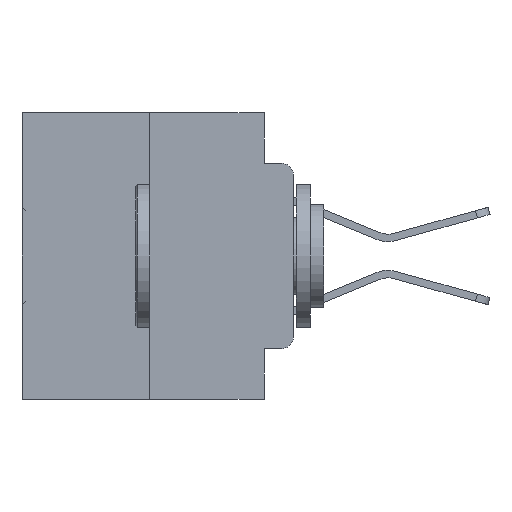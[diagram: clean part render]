
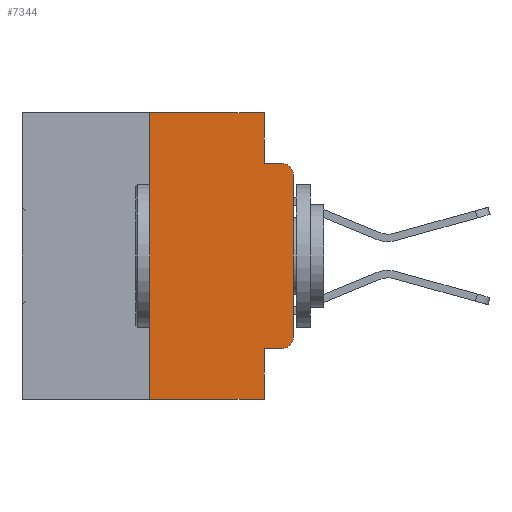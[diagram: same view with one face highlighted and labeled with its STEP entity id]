
A CAD part, left-side view. The second image highlights one B-rep face of the part: STEP entity #7344.
In plain terms, the highlighted planar face has unit normal (-1, 0, 0).
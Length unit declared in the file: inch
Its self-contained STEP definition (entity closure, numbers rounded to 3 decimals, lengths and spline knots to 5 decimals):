
#175 = EDGE_CURVE ( 'NONE', #24864, #2652, #18759, .T. ) ;
#253 = EDGE_CURVE ( 'NONE', #2652, #20397, #9630, .T. ) ;
#438 = CARTESIAN_POINT ( 'NONE',  ( 0., 0.051, -0.0885 ) ) ;
#576 = CARTESIAN_POINT ( 'NONE',  ( 0., 0.051, 0. ) ) ;
#759 = PLANE ( 'NONE',  #2581 ) ;
#1670 = VERTEX_POINT ( 'NONE', #30321 ) ;
#1920 = ORIENTED_EDGE ( 'NONE', *, *, #18589, .T. ) ;
#2013 = DIRECTION ( 'NONE',  ( 0., 0., -1. ) ) ;
#2068 = CARTESIAN_POINT ( 'NONE',  ( 0., 0.25, 0. ) ) ;
#2276 = CARTESIAN_POINT ( 'NONE',  ( 0., 0.02, -0.4115 ) ) ;
#2544 = VECTOR ( 'NONE', #8177, 39.37008 ) ;
#2581 = AXIS2_PLACEMENT_3D ( 'NONE', #8511, #15895, #5812 ) ;
#2652 = VERTEX_POINT ( 'NONE', #10949 ) ;
#3307 = VECTOR ( 'NONE', #26585, 39.37008 ) ;
#4501 = VERTEX_POINT ( 'NONE', #12056 ) ;
#4738 = VECTOR ( 'NONE', #5002, 39.37008 ) ;
#4753 = EDGE_CURVE ( 'NONE', #4501, #22494, #8664, .T. ) ;
#5002 = DIRECTION ( 'NONE',  ( 0., -1., 0. ) ) ;
#5324 = LINE ( 'NONE', #15572, #4738 ) ;
#5365 = DIRECTION ( 'NONE',  ( 0., -1., 0. ) ) ;
#5481 = CARTESIAN_POINT ( 'NONE',  ( 0., 0.051, -0.4115 ) ) ;
#5764 = LINE ( 'NONE', #31781, #31315 ) ;
#5812 = DIRECTION ( 'NONE',  ( 0., 0., -1. ) ) ;
#6487 = CARTESIAN_POINT ( 'NONE',  ( 0., 0.25, 0. ) ) ;
#7344 = ADVANCED_FACE ( 'NONE', ( #28811 ), #759, .F. ) ;
#7726 = EDGE_CURVE ( 'NONE', #24086, #4501, #5324, .T. ) ;
#8177 = DIRECTION ( 'NONE',  ( 0., 0., 1. ) ) ;
#8352 = CARTESIAN_POINT ( 'NONE',  ( 0., 0., 0. ) ) ;
#8430 = CARTESIAN_POINT ( 'NONE',  ( 0., 0.02, -0.0885 ) ) ;
#8511 = CARTESIAN_POINT ( 'NONE',  ( 0., 0.473, 0. ) ) ;
#8664 = LINE ( 'NONE', #576, #22919 ) ;
#9367 = DIRECTION ( 'NONE',  ( 0., 0., -1. ) ) ;
#9630 = CIRCLE ( 'NONE', #31566, 0.02 ) ;
#9819 = VECTOR ( 'NONE', #5365, 39.37008 ) ;
#10439 = LINE ( 'NONE', #13259, #24296 ) ;
#10949 = CARTESIAN_POINT ( 'NONE',  ( 0., 0., -0.1085 ) ) ;
#11005 = DIRECTION ( 'NONE',  ( 0., 0., -1. ) ) ;
#11677 = DIRECTION ( 'NONE',  ( 0., 0., 1. ) ) ;
#11937 = VERTEX_POINT ( 'NONE', #5481 ) ;
#12056 = CARTESIAN_POINT ( 'NONE',  ( 0., 0.051, 0. ) ) ;
#12322 = CARTESIAN_POINT ( 'NONE',  ( 0., 0., -0.3915 ) ) ;
#12771 = DIRECTION ( 'NONE',  ( 0., -1., 0. ) ) ;
#13259 = CARTESIAN_POINT ( 'NONE',  ( 0., 0.051, -0.4115 ) ) ;
#13326 = ORIENTED_EDGE ( 'NONE', *, *, #7726, .F. ) ;
#13506 = LINE ( 'NONE', #31626, #3307 ) ;
#14018 = EDGE_CURVE ( 'NONE', #19169, #24086, #22564, .T. ) ;
#14299 = DIRECTION ( 'NONE',  ( -1., 0., 0. ) ) ;
#15572 = CARTESIAN_POINT ( 'NONE',  ( 0., 0.473, 0. ) ) ;
#15895 = DIRECTION ( 'NONE',  ( 1., 0., 0. ) ) ;
#16673 = EDGE_CURVE ( 'NONE', #11937, #1670, #5764, .T. ) ;
#17281 = EDGE_LOOP ( 'NONE', ( #30604, #31791, #18895, #23399, #13326, #21141, #28753, #22135, #27147, #1920 ) ) ;
#18476 = LINE ( 'NONE', #26006, #9819 ) ;
#18589 = EDGE_CURVE ( 'NONE', #22870, #24864, #28412, .T. ) ;
#18759 = LINE ( 'NONE', #8352, #2544 ) ;
#18895 = ORIENTED_EDGE ( 'NONE', *, *, #32709, .F. ) ;
#19169 = VERTEX_POINT ( 'NONE', #20621 ) ;
#20397 = VERTEX_POINT ( 'NONE', #8430 ) ;
#20621 = CARTESIAN_POINT ( 'NONE',  ( 0., 0.25, -0.5 ) ) ;
#21141 = ORIENTED_EDGE ( 'NONE', *, *, #14018, .F. ) ;
#22034 = EDGE_CURVE ( 'NONE', #11937, #22870, #10439, .T. ) ;
#22135 = ORIENTED_EDGE ( 'NONE', *, *, #16673, .F. ) ;
#22494 = VERTEX_POINT ( 'NONE', #438 ) ;
#22564 = LINE ( 'NONE', #2068, #25795 ) ;
#22870 = VERTEX_POINT ( 'NONE', #2276 ) ;
#22919 = VECTOR ( 'NONE', #31142, 39.37008 ) ;
#23399 = ORIENTED_EDGE ( 'NONE', *, *, #4753, .F. ) ;
#24086 = VERTEX_POINT ( 'NONE', #6487 ) ;
#24296 = VECTOR ( 'NONE', #12771, 39.37008 ) ;
#24864 = VERTEX_POINT ( 'NONE', #12322 ) ;
#25795 = VECTOR ( 'NONE', #11677, 39.37008 ) ;
#26006 = CARTESIAN_POINT ( 'NONE',  ( 0., 0.051, -0.0885 ) ) ;
#26585 = DIRECTION ( 'NONE',  ( 0., -1., 0. ) ) ;
#26782 = DIRECTION ( 'NONE',  ( -1., 0., 0. ) ) ;
#27147 = ORIENTED_EDGE ( 'NONE', *, *, #22034, .T. ) ;
#28412 = CIRCLE ( 'NONE', #29470, 0.02 ) ;
#28753 = ORIENTED_EDGE ( 'NONE', *, *, #31816, .T. ) ;
#28811 = FACE_OUTER_BOUND ( 'NONE', #17281, .T. ) ;
#29470 = AXIS2_PLACEMENT_3D ( 'NONE', #32582, #14299, #2013 ) ;
#30321 = CARTESIAN_POINT ( 'NONE',  ( 0., 0.051, -0.5 ) ) ;
#30604 = ORIENTED_EDGE ( 'NONE', *, *, #175, .T. ) ;
#31142 = DIRECTION ( 'NONE',  ( 0., 0., -1. ) ) ;
#31315 = VECTOR ( 'NONE', #11005, 39.37008 ) ;
#31566 = AXIS2_PLACEMENT_3D ( 'NONE', #32335, #26782, #9367 ) ;
#31626 = CARTESIAN_POINT ( 'NONE',  ( 0., 0.473, -0.5 ) ) ;
#31781 = CARTESIAN_POINT ( 'NONE',  ( 0., 0.051, 0. ) ) ;
#31791 = ORIENTED_EDGE ( 'NONE', *, *, #253, .T. ) ;
#31816 = EDGE_CURVE ( 'NONE', #19169, #1670, #13506, .T. ) ;
#32335 = CARTESIAN_POINT ( 'NONE',  ( 0., 0.02, -0.1085 ) ) ;
#32582 = CARTESIAN_POINT ( 'NONE',  ( 0., 0.02, -0.3915 ) ) ;
#32709 = EDGE_CURVE ( 'NONE', #22494, #20397, #18476, .T. ) ;
